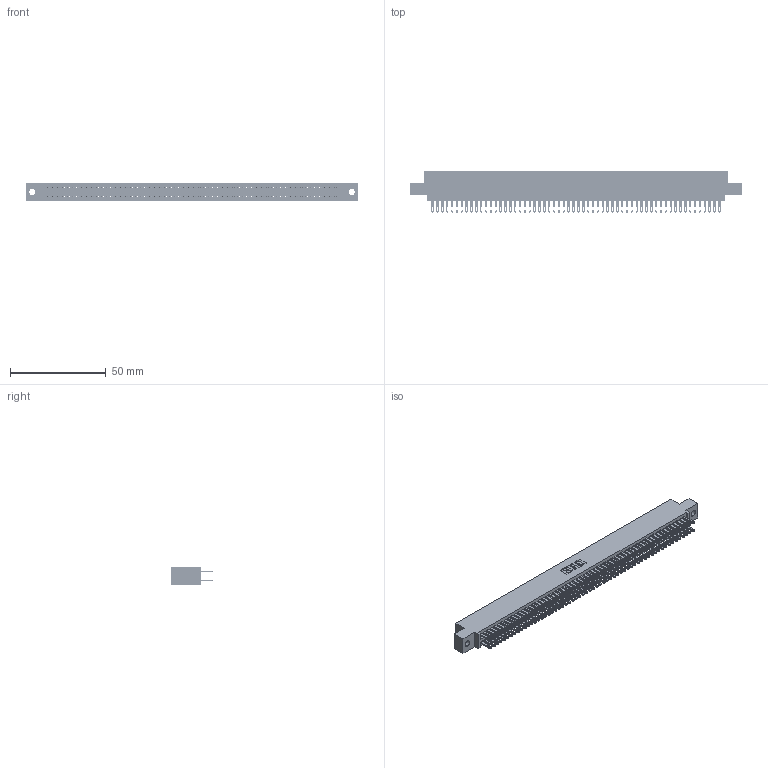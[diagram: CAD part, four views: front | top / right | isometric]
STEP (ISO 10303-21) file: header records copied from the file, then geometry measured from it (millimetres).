
FILE_DESCRIPTION (( 'STEP AP203' ), '1' );
FILE_NAME ('895-120-500-502.STEP', '2020-10-13T14:58:58', ( '' ), ( '' ), 'SwSTEP 2.0', 'SolidWorks 2020', '' );
FILE_SCHEMA (( 'CONFIG_CONTROL_DESIGN' ));
Length unit declared in the file: inch
Products named in the file (3): 345-292-001_345-293-100; 845 Part_0.110 Offset - 0.128 Dia; 895-120-500-502
Assembly tree (121 placements, depth 2):
  895-120-500-502
    845 Part_0.110 Offset - 0.128 Dia
    345-292-001_345-293-100  x120
Bounding box: 173.61 x 21.51 x 9.4 mm (x, y, z)
Volume: 17288.3 mm3; surface area: 26947.7 mm2
Topology: 121 solids, 121 shells, 5650 faces, 17273 edges, 11514 vertices
Faces by surface type: plane 3324, cylinder 2326
Entity records: 44719 total; most frequent: CARTESIAN_POINT 7480, ORIENTED_EDGE 7414, DIRECTION 6575, EDGE_CURVE 3707, VECTOR 3331, LINE 3331, VERTEX_POINT 2470, AXIS2_PLACEMENT_3D 1622
